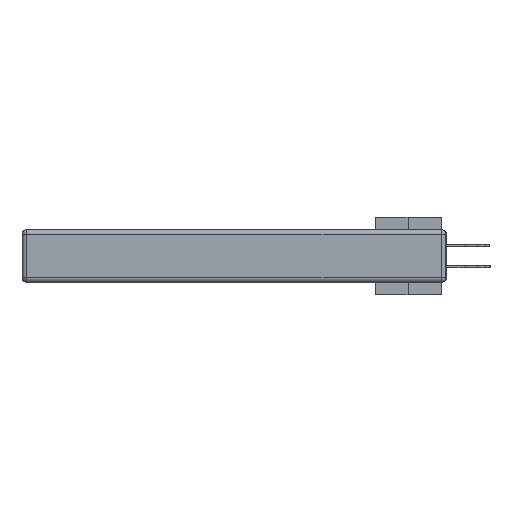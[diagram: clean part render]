
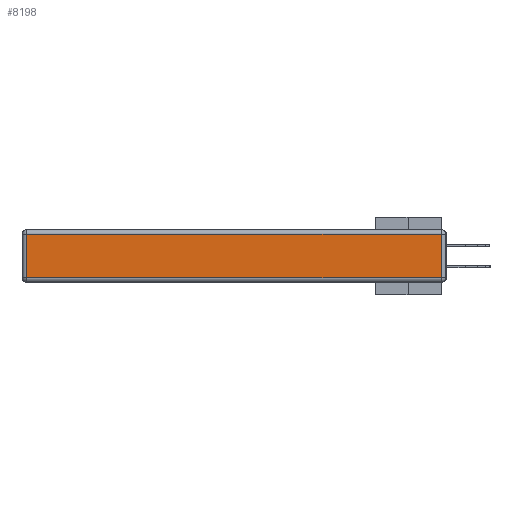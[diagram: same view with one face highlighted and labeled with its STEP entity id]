
A CAD part, left-side view. The second image highlights one B-rep face of the part: STEP entity #8198.
In plain terms, the highlighted planar face has unit normal (-1, 0, 0).
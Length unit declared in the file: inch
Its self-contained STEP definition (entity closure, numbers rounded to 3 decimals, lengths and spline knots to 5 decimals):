
#1018 = CARTESIAN_POINT ( 'NONE',  ( 0., 2.72, -0.343 ) ) ;
#1449 = DIRECTION ( 'NONE',  ( -1., 0., 0. ) ) ;
#4279 = ORIENTED_EDGE ( 'NONE', *, *, #9848, .T. ) ;
#4602 = DIRECTION ( 'NONE',  ( 0., 0., 1. ) ) ;
#5072 = VECTOR ( 'NONE', #10590, 39.37008 ) ;
#5283 = EDGE_CURVE ( 'NONE', #38098, #18654, #11388, .T. ) ;
#5359 = DIRECTION ( 'NONE',  ( 0., 1., 0. ) ) ;
#6311 = CARTESIAN_POINT ( 'NONE',  ( 0., 2.72, -0.313 ) ) ;
#6470 = ORIENTED_EDGE ( 'NONE', *, *, #10831, .T. ) ;
#8198 = ADVANCED_FACE ( 'NONE', ( #11459 ), #10879, .T. ) ;
#9848 = EDGE_CURVE ( 'NONE', #14057, #17471, #31980, .T. ) ;
#10590 = DIRECTION ( 'NONE',  ( 0., 0., -1. ) ) ;
#10831 = EDGE_CURVE ( 'NONE', #17471, #38098, #22100, .T. ) ;
#10879 = PLANE ( 'NONE',  #34642 ) ;
#10971 = DIRECTION ( 'NONE',  ( 0., -1., 0. ) ) ;
#10988 = EDGE_CURVE ( 'NONE', #18654, #14057, #18696, .T. ) ;
#11388 = LINE ( 'NONE', #17642, #31968 ) ;
#11459 = FACE_OUTER_BOUND ( 'NONE', #38870, .T. ) ;
#14057 = VERTEX_POINT ( 'NONE', #24433 ) ;
#14106 = DIRECTION ( 'NONE',  ( 0., 0., 1. ) ) ;
#14744 = VECTOR ( 'NONE', #10971, 39.37008 ) ;
#17471 = VERTEX_POINT ( 'NONE', #6311 ) ;
#17642 = CARTESIAN_POINT ( 'NONE',  ( 0., 0.03, -0.343 ) ) ;
#17690 = CARTESIAN_POINT ( 'NONE',  ( 0., 0.03, -0.313 ) ) ;
#18654 = VERTEX_POINT ( 'NONE', #29866 ) ;
#18696 = LINE ( 'NONE', #30503, #34343 ) ;
#20193 = CARTESIAN_POINT ( 'NONE',  ( 0., 0., -0.343 ) ) ;
#21069 = ORIENTED_EDGE ( 'NONE', *, *, #5283, .T. ) ;
#22100 = LINE ( 'NONE', #23822, #14744 ) ;
#23822 = CARTESIAN_POINT ( 'NONE',  ( 0., 0., -0.313 ) ) ;
#24433 = CARTESIAN_POINT ( 'NONE',  ( 0., 2.72, -0.03 ) ) ;
#24535 = ORIENTED_EDGE ( 'NONE', *, *, #10988, .T. ) ;
#29866 = CARTESIAN_POINT ( 'NONE',  ( 0., 0.03, -0.03 ) ) ;
#30503 = CARTESIAN_POINT ( 'NONE',  ( 0., 2.75, -0.03 ) ) ;
#31968 = VECTOR ( 'NONE', #14106, 39.37008 ) ;
#31980 = LINE ( 'NONE', #1018, #5072 ) ;
#34343 = VECTOR ( 'NONE', #5359, 39.37008 ) ;
#34642 = AXIS2_PLACEMENT_3D ( 'NONE', #20193, #1449, #4602 ) ;
#38098 = VERTEX_POINT ( 'NONE', #17690 ) ;
#38870 = EDGE_LOOP ( 'NONE', ( #6470, #21069, #24535, #4279 ) ) ;
